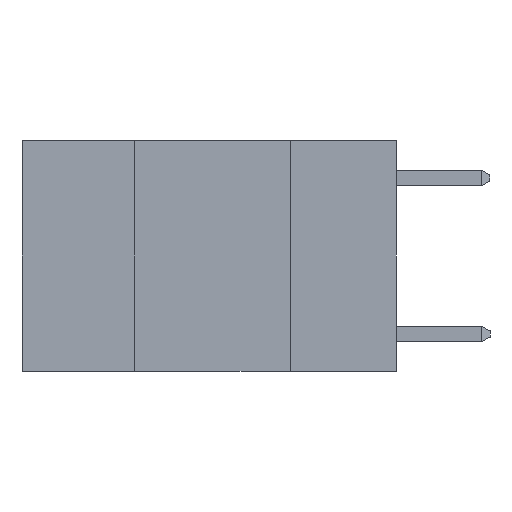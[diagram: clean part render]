
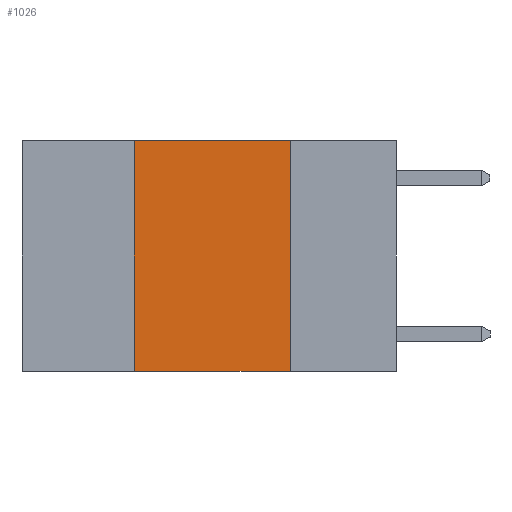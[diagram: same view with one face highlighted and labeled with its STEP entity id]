
A CAD part, left-side view. The second image highlights one B-rep face of the part: STEP entity #1026.
In plain terms, the highlighted planar face has unit normal (-1, 0, 0).
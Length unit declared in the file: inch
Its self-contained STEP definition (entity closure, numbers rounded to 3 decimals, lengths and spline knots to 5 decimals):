
#119 = CARTESIAN_POINT ( 'NONE',  ( 0., 0.6, 0. ) ) ;
#845 = DIRECTION ( 'NONE',  ( 0., -1., 0. ) ) ;
#879 = VERTEX_POINT ( 'NONE', #8134 ) ;
#896 = ORIENTED_EDGE ( 'NONE', *, *, #4119, .F. ) ;
#1026 = ADVANCED_FACE ( 'NONE', ( #5725 ), #7420, .F. ) ;
#1053 = AXIS2_PLACEMENT_3D ( 'NONE', #7703, #5480, #1188 ) ;
#1175 = ORIENTED_EDGE ( 'NONE', *, *, #8058, .F. ) ;
#1188 = DIRECTION ( 'NONE',  ( 0., 0., -1. ) ) ;
#1209 = CARTESIAN_POINT ( 'NONE',  ( 0., 0.17, 0. ) ) ;
#1426 = LINE ( 'NONE', #1209, #6625 ) ;
#2045 = LINE ( 'NONE', #7439, #5647 ) ;
#2103 = CARTESIAN_POINT ( 'NONE',  ( 0., 0.17, 0. ) ) ;
#2128 = ORIENTED_EDGE ( 'NONE', *, *, #8681, .T. ) ;
#2370 = VECTOR ( 'NONE', #7361, 39.37008 ) ;
#2405 = LINE ( 'NONE', #119, #7572 ) ;
#2957 = EDGE_LOOP ( 'NONE', ( #1175, #896, #6710, #2128 ) ) ;
#3261 = DIRECTION ( 'NONE',  ( 0., 0., -1. ) ) ;
#4119 = EDGE_CURVE ( 'NONE', #879, #5201, #2405, .T. ) ;
#4185 = CARTESIAN_POINT ( 'NONE',  ( 0., 0.17, -0.37 ) ) ;
#4360 = CARTESIAN_POINT ( 'NONE',  ( 0., 0.42, -0.37 ) ) ;
#4773 = VERTEX_POINT ( 'NONE', #4185 ) ;
#5201 = VERTEX_POINT ( 'NONE', #2103 ) ;
#5480 = DIRECTION ( 'NONE',  ( 1., 0., 0. ) ) ;
#5647 = VECTOR ( 'NONE', #8091, 39.37008 ) ;
#5725 = FACE_OUTER_BOUND ( 'NONE', #2957, .T. ) ;
#5753 = LINE ( 'NONE', #6694, #2370 ) ;
#5767 = EDGE_CURVE ( 'NONE', #6800, #879, #2045, .T. ) ;
#6625 = VECTOR ( 'NONE', #3261, 39.37008 ) ;
#6694 = CARTESIAN_POINT ( 'NONE',  ( 0., 0.6, -0.37 ) ) ;
#6710 = ORIENTED_EDGE ( 'NONE', *, *, #5767, .F. ) ;
#6800 = VERTEX_POINT ( 'NONE', #4360 ) ;
#7361 = DIRECTION ( 'NONE',  ( 0., -1., 0. ) ) ;
#7420 = PLANE ( 'NONE',  #1053 ) ;
#7439 = CARTESIAN_POINT ( 'NONE',  ( 0., 0.42, 0. ) ) ;
#7572 = VECTOR ( 'NONE', #845, 39.37008 ) ;
#7703 = CARTESIAN_POINT ( 'NONE',  ( 0., 0.6, 0. ) ) ;
#8058 = EDGE_CURVE ( 'NONE', #5201, #4773, #1426, .T. ) ;
#8091 = DIRECTION ( 'NONE',  ( 0., 0., 1. ) ) ;
#8134 = CARTESIAN_POINT ( 'NONE',  ( 0., 0.42, 0. ) ) ;
#8681 = EDGE_CURVE ( 'NONE', #6800, #4773, #5753, .T. ) ;
